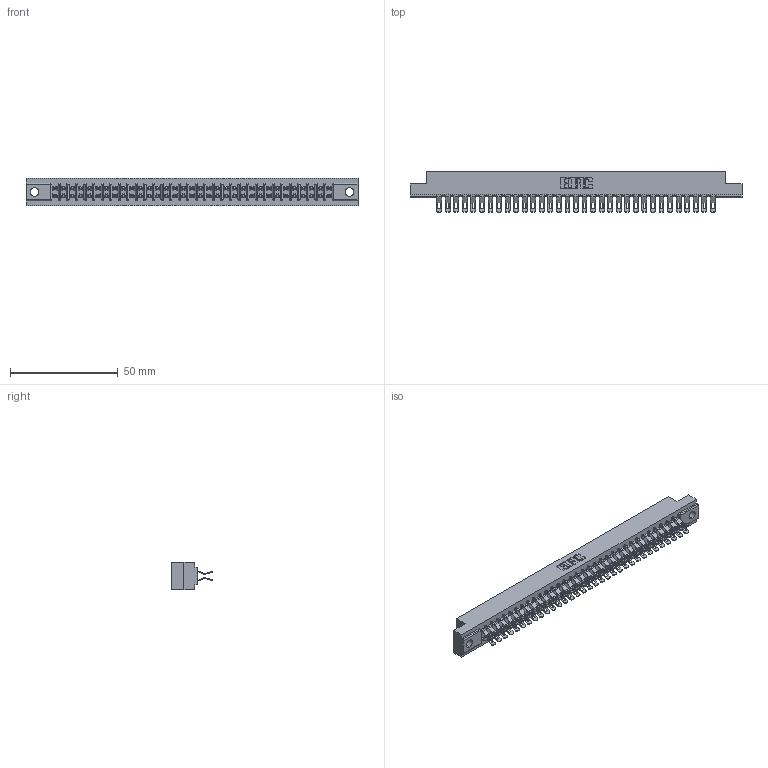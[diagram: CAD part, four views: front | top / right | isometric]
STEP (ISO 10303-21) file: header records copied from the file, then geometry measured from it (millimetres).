
FILE_DESCRIPTION (( 'STEP AP203' ), '1' );
FILE_NAME ('357-066-555-202.STEP', '2019-09-19T08:44:32', ( '' ), ( '' ), 'SwSTEP 2.0', 'SolidWorks 2016', '' );
FILE_SCHEMA (( 'CONFIG_CONTROL_DESIGN' ));
Length unit declared in the file: inch
Products named in the file (3): 307 Part_.128 Dia Mounting Holes; 357-066-555-202; 307-290-001_555
Assembly tree (67 placements, depth 2):
  357-066-555-202
    307 Part_.128 Dia Mounting Holes
    307-290-001_555  x66
Bounding box: 153.77 x 18.75 x 12.7 mm (x, y, z)
Volume: 16396.8 mm3; surface area: 20773.8 mm2
Topology: 67 solids, 67 shells, 4178 faces, 12269 edges, 7998 vertices
Faces by surface type: plane 2314, cylinder 1796, sphere 68
Entity records: 30995 total; most frequent: CARTESIAN_POINT 5077, ORIENTED_EDGE 5032, DIRECTION 4984, EDGE_CURVE 2516, LINE 1914, VECTOR 1914, VERTEX_POINT 1628, AXIS2_PLACEMENT_3D 1535
